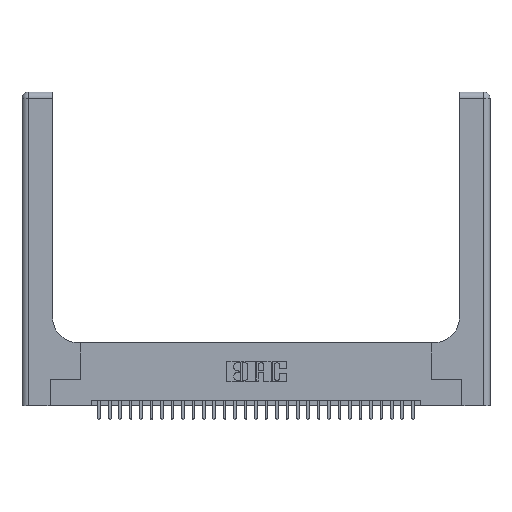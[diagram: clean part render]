
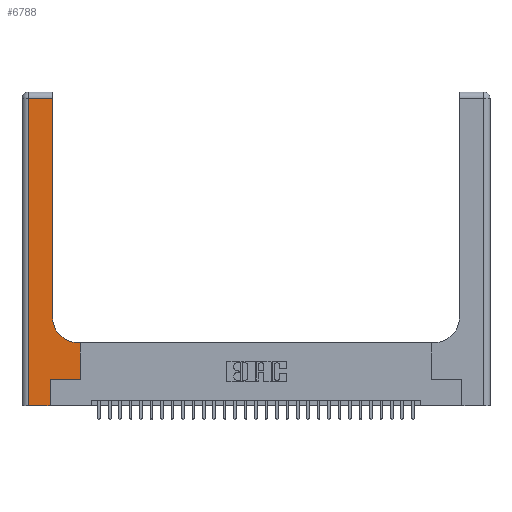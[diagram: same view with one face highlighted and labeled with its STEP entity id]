
A CAD part, top view. The second image highlights one B-rep face of the part: STEP entity #6788.
In plain terms, the highlighted planar face has unit normal (0, 0, 1).
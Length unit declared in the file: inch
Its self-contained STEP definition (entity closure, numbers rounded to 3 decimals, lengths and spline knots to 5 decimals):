
#395 = VECTOR ( 'NONE', #16649, 39.37008 ) ;
#482 = ORIENTED_EDGE ( 'NONE', *, *, #17785, .T. ) ;
#533 = ORIENTED_EDGE ( 'NONE', *, *, #22506, .T. ) ;
#627 = CARTESIAN_POINT ( 'NONE',  ( 0.2915, 3., 0.37 ) ) ;
#952 = EDGE_CURVE ( 'NONE', #7039, #19891, #17130, .T. ) ;
#1036 = VERTEX_POINT ( 'NONE', #13625 ) ;
#1528 = ORIENTED_EDGE ( 'NONE', *, *, #21493, .T. ) ;
#2056 = VECTOR ( 'NONE', #8290, 39.37008 ) ;
#2348 = CARTESIAN_POINT ( 'NONE',  ( 0.5415, 0.85, 0.37 ) ) ;
#3376 = CARTESIAN_POINT ( 'NONE',  ( 0.5585, 0.25, 0.37 ) ) ;
#3393 = CARTESIAN_POINT ( 'NONE',  ( 0.5415, 0.6, 0.37 ) ) ;
#4326 = CARTESIAN_POINT ( 'NONE',  ( 0.269, 0.25, 0.37 ) ) ;
#4808 = CARTESIAN_POINT ( 'NONE',  ( 0.2915, 0.85, 0.37 ) ) ;
#4902 = LINE ( 'NONE', #19305, #395 ) ;
#6320 = CARTESIAN_POINT ( 'NONE',  ( 0.06, 0., 0.37 ) ) ;
#6455 = CIRCLE ( 'NONE', #17040, 0.25 ) ;
#6788 = ADVANCED_FACE ( 'NONE', ( #13328 ), #7989, .F. ) ;
#7039 = VERTEX_POINT ( 'NONE', #27324 ) ;
#7986 = LINE ( 'NONE', #21547, #9856 ) ;
#7989 = PLANE ( 'NONE',  #30109 ) ;
#8235 = VERTEX_POINT ( 'NONE', #6320 ) ;
#8290 = DIRECTION ( 'NONE',  ( 0., -1., 0. ) ) ;
#9251 = DIRECTION ( 'NONE',  ( 1., 0., 0. ) ) ;
#9566 = DIRECTION ( 'NONE',  ( 1., 0., 0. ) ) ;
#9796 = VERTEX_POINT ( 'NONE', #29576 ) ;
#9856 = VECTOR ( 'NONE', #26483, 39.37008 ) ;
#9969 = ORIENTED_EDGE ( 'NONE', *, *, #16254, .T. ) ;
#10303 = CARTESIAN_POINT ( 'NONE',  ( 0., 3., 0.37 ) ) ;
#10680 = EDGE_CURVE ( 'NONE', #1036, #24022, #17490, .T. ) ;
#10723 = CARTESIAN_POINT ( 'NONE',  ( 0.5585, 0.25, 0.37 ) ) ;
#10791 = CARTESIAN_POINT ( 'NONE',  ( 0.06, 3., 0.37 ) ) ;
#11128 = VECTOR ( 'NONE', #9251, 39.37008 ) ;
#11905 = EDGE_CURVE ( 'NONE', #9796, #8235, #23431, .T. ) ;
#12262 = VECTOR ( 'NONE', #19568, 39.37008 ) ;
#13328 = FACE_OUTER_BOUND ( 'NONE', #16086, .T. ) ;
#13437 = LINE ( 'NONE', #627, #12262 ) ;
#13561 = CARTESIAN_POINT ( 'NONE',  ( 0.2915, 0.6, 0.37 ) ) ;
#13614 = CARTESIAN_POINT ( 'NONE',  ( 0.269, 0., 0.37 ) ) ;
#13625 = CARTESIAN_POINT ( 'NONE',  ( 0.269, 0.25, 0.37 ) ) ;
#14054 = ORIENTED_EDGE ( 'NONE', *, *, #20549, .T. ) ;
#14735 = ORIENTED_EDGE ( 'NONE', *, *, #952, .T. ) ;
#14968 = VECTOR ( 'NONE', #24895, 39.37008 ) ;
#15035 = DIRECTION ( 'NONE',  ( 0., 0., -1. ) ) ;
#15427 = VERTEX_POINT ( 'NONE', #30088 ) ;
#16086 = EDGE_LOOP ( 'NONE', ( #533, #1528, #30871, #482, #27118, #30716, #14054, #14735, #9969 ) ) ;
#16254 = EDGE_CURVE ( 'NONE', #19891, #27436, #6455, .T. ) ;
#16649 = DIRECTION ( 'NONE',  ( 0., 1., 0. ) ) ;
#16859 = EDGE_CURVE ( 'NONE', #21107, #1036, #4902, .T. ) ;
#17040 = AXIS2_PLACEMENT_3D ( 'NONE', #2348, #23942, #9566 ) ;
#17130 = LINE ( 'NONE', #13561, #17514 ) ;
#17490 = LINE ( 'NONE', #4326, #11128 ) ;
#17514 = VECTOR ( 'NONE', #30284, 39.37008 ) ;
#17785 = EDGE_CURVE ( 'NONE', #8235, #21107, #28083, .T. ) ;
#17962 = DIRECTION ( 'NONE',  ( 0., 1., 0. ) ) ;
#19305 = CARTESIAN_POINT ( 'NONE',  ( 0.269, 0., 0.37 ) ) ;
#19568 = DIRECTION ( 'NONE',  ( 0., 1., 0. ) ) ;
#19891 = VERTEX_POINT ( 'NONE', #3393 ) ;
#20523 = VECTOR ( 'NONE', #17962, 39.37008 ) ;
#20549 = EDGE_CURVE ( 'NONE', #24022, #7039, #27541, .T. ) ;
#21107 = VERTEX_POINT ( 'NONE', #13614 ) ;
#21493 = EDGE_CURVE ( 'NONE', #15427, #9796, #7986, .T. ) ;
#21547 = CARTESIAN_POINT ( 'NONE',  ( 0., 2.94, 0.37 ) ) ;
#22506 = EDGE_CURVE ( 'NONE', #27436, #15427, #13437, .T. ) ;
#23431 = LINE ( 'NONE', #10791, #2056 ) ;
#23942 = DIRECTION ( 'NONE',  ( 0., 0., -1. ) ) ;
#24022 = VERTEX_POINT ( 'NONE', #10723 ) ;
#24895 = DIRECTION ( 'NONE',  ( 1., 0., 0. ) ) ;
#25207 = CARTESIAN_POINT ( 'NONE',  ( 0., 0., 0.37 ) ) ;
#26483 = DIRECTION ( 'NONE',  ( -1., 0., 0. ) ) ;
#27118 = ORIENTED_EDGE ( 'NONE', *, *, #16859, .T. ) ;
#27324 = CARTESIAN_POINT ( 'NONE',  ( 0.5585, 0.6, 0.37 ) ) ;
#27436 = VERTEX_POINT ( 'NONE', #4808 ) ;
#27541 = LINE ( 'NONE', #3376, #20523 ) ;
#28083 = LINE ( 'NONE', #25207, #14968 ) ;
#29570 = DIRECTION ( 'NONE',  ( -1., 0., 0. ) ) ;
#29576 = CARTESIAN_POINT ( 'NONE',  ( 0.06, 2.94, 0.37 ) ) ;
#30088 = CARTESIAN_POINT ( 'NONE',  ( 0.2915, 2.94, 0.37 ) ) ;
#30109 = AXIS2_PLACEMENT_3D ( 'NONE', #10303, #15035, #29570 ) ;
#30284 = DIRECTION ( 'NONE',  ( -1., 0., 0. ) ) ;
#30716 = ORIENTED_EDGE ( 'NONE', *, *, #10680, .T. ) ;
#30871 = ORIENTED_EDGE ( 'NONE', *, *, #11905, .T. ) ;
